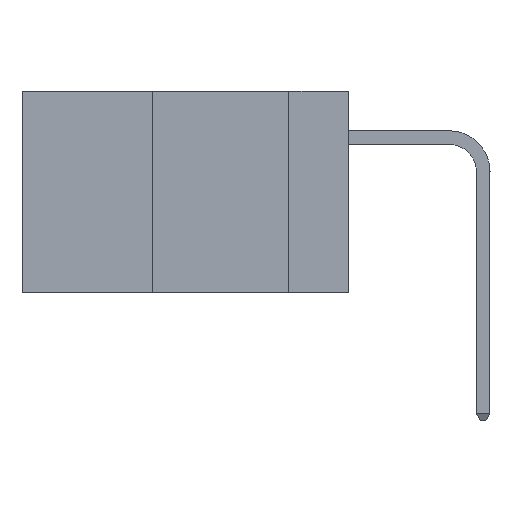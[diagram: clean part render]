
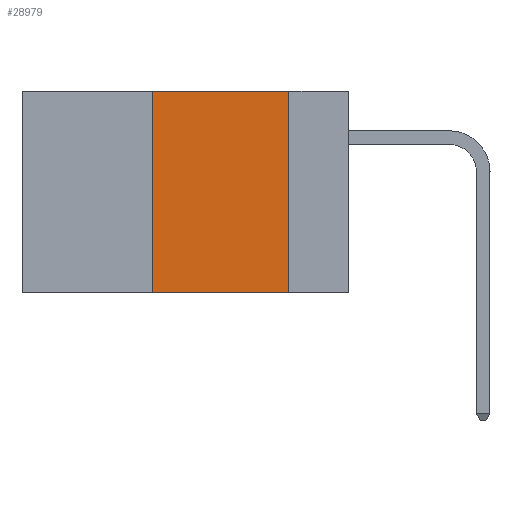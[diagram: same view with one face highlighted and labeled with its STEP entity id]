
A CAD part, left-side view. The second image highlights one B-rep face of the part: STEP entity #28979.
In plain terms, the highlighted planar face has unit normal (-1, 0, 0).
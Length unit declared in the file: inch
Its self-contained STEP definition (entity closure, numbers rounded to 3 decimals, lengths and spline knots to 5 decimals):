
#2404 = PLANE ( 'NONE',  #42897 ) ;
#2559 = ORIENTED_EDGE ( 'NONE', *, *, #31975, .F. ) ;
#3530 = VECTOR ( 'NONE', #30629, 39.37008 ) ;
#5784 = LINE ( 'NONE', #26790, #30505 ) ;
#7453 = CARTESIAN_POINT ( 'NONE',  ( 0., 0.36, -0.37 ) ) ;
#9776 = EDGE_CURVE ( 'NONE', #38264, #16326, #39254, .T. ) ;
#11221 = CARTESIAN_POINT ( 'NONE',  ( 0., 0.36, 0. ) ) ;
#12315 = CARTESIAN_POINT ( 'NONE',  ( 0., 0.6, 0. ) ) ;
#13362 = DIRECTION ( 'NONE',  ( 0., 0., -1. ) ) ;
#14938 = CARTESIAN_POINT ( 'NONE',  ( 0., 0.11, -0.37 ) ) ;
#15787 = ORIENTED_EDGE ( 'NONE', *, *, #9776, .T. ) ;
#16036 = VERTEX_POINT ( 'NONE', #16902 ) ;
#16326 = VERTEX_POINT ( 'NONE', #14938 ) ;
#16902 = CARTESIAN_POINT ( 'NONE',  ( 0., 0.11, 0. ) ) ;
#18242 = EDGE_CURVE ( 'NONE', #34679, #16036, #20352, .T. ) ;
#19200 = EDGE_LOOP ( 'NONE', ( #23958, #43509, #2559, #15787 ) ) ;
#19345 = DIRECTION ( 'NONE',  ( 1., 0., 0. ) ) ;
#19744 = DIRECTION ( 'NONE',  ( 0., 0., 1. ) ) ;
#20352 = LINE ( 'NONE', #12315, #29251 ) ;
#21097 = VECTOR ( 'NONE', #19744, 39.37008 ) ;
#22569 = EDGE_CURVE ( 'NONE', #16036, #16326, #5784, .T. ) ;
#23958 = ORIENTED_EDGE ( 'NONE', *, *, #22569, .F. ) ;
#26790 = CARTESIAN_POINT ( 'NONE',  ( 0., 0.11, 0. ) ) ;
#27279 = CARTESIAN_POINT ( 'NONE',  ( 0., 0.6, -0.37 ) ) ;
#28979 = ADVANCED_FACE ( 'NONE', ( #39710 ), #2404, .F. ) ;
#29251 = VECTOR ( 'NONE', #35817, 39.37008 ) ;
#30505 = VECTOR ( 'NONE', #13362, 39.37008 ) ;
#30629 = DIRECTION ( 'NONE',  ( 0., -1., 0. ) ) ;
#31975 = EDGE_CURVE ( 'NONE', #38264, #34679, #37836, .T. ) ;
#34679 = VERTEX_POINT ( 'NONE', #11221 ) ;
#35817 = DIRECTION ( 'NONE',  ( 0., -1., 0. ) ) ;
#37836 = LINE ( 'NONE', #43136, #21097 ) ;
#38264 = VERTEX_POINT ( 'NONE', #7453 ) ;
#39254 = LINE ( 'NONE', #27279, #3530 ) ;
#39429 = CARTESIAN_POINT ( 'NONE',  ( 0., 0.6, 0. ) ) ;
#39710 = FACE_OUTER_BOUND ( 'NONE', #19200, .T. ) ;
#42763 = DIRECTION ( 'NONE',  ( 0., 0., -1. ) ) ;
#42897 = AXIS2_PLACEMENT_3D ( 'NONE', #39429, #19345, #42763 ) ;
#43136 = CARTESIAN_POINT ( 'NONE',  ( 0., 0.36, 0. ) ) ;
#43509 = ORIENTED_EDGE ( 'NONE', *, *, #18242, .F. ) ;
